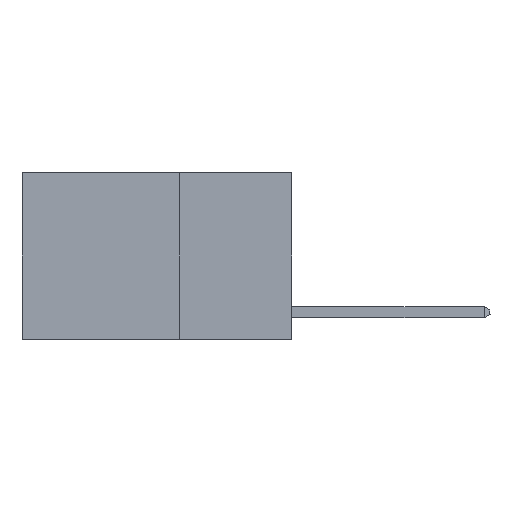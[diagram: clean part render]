
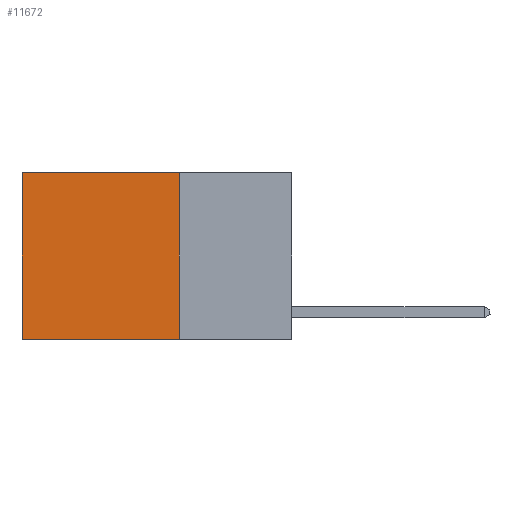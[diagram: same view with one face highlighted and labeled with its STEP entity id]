
A CAD part, left-side view. The second image highlights one B-rep face of the part: STEP entity #11672.
In plain terms, the highlighted planar face has unit normal (-1, 0, 0).
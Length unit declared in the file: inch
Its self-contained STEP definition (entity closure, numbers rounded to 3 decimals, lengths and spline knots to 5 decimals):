
#360 = VECTOR ( 'NONE', #8419, 39.37008 ) ;
#2024 = ORIENTED_EDGE ( 'NONE', *, *, #18143, .T. ) ;
#2514 = CARTESIAN_POINT ( 'NONE',  ( 0.2625, 0.6, -0.37 ) ) ;
#2698 = EDGE_LOOP ( 'NONE', ( #2024, #26090, #4861, #4713 ) ) ;
#2784 = VECTOR ( 'NONE', #22954, 39.37008 ) ;
#2805 = DIRECTION ( 'NONE',  ( 0., 0., -1. ) ) ;
#3324 = LINE ( 'NONE', #10023, #9294 ) ;
#4713 = ORIENTED_EDGE ( 'NONE', *, *, #6314, .T. ) ;
#4786 = VERTEX_POINT ( 'NONE', #8839 ) ;
#4861 = ORIENTED_EDGE ( 'NONE', *, *, #15027, .F. ) ;
#5280 = EDGE_CURVE ( 'NONE', #4786, #11597, #12227, .T. ) ;
#5562 = DIRECTION ( 'NONE',  ( 0., 0., -1. ) ) ;
#6314 = EDGE_CURVE ( 'NONE', #15035, #21700, #15975, .T. ) ;
#7137 = CARTESIAN_POINT ( 'NONE',  ( 0.2625, 0.6, 0. ) ) ;
#8419 = DIRECTION ( 'NONE',  ( 0., 1., 0. ) ) ;
#8839 = CARTESIAN_POINT ( 'NONE',  ( 0.2625, 0.25, -0.37 ) ) ;
#9294 = VECTOR ( 'NONE', #5562, 39.37008 ) ;
#10023 = CARTESIAN_POINT ( 'NONE',  ( 0.2625, 0.25, 0. ) ) ;
#10555 = CARTESIAN_POINT ( 'NONE',  ( 0.2625, 0.25, -0.37 ) ) ;
#11597 = VERTEX_POINT ( 'NONE', #2514 ) ;
#11658 = PLANE ( 'NONE',  #14629 ) ;
#11672 = ADVANCED_FACE ( 'NONE', ( #21176 ), #11658, .F. ) ;
#12227 = LINE ( 'NONE', #10555, #360 ) ;
#13778 = DIRECTION ( 'NONE',  ( 0., 0., -1. ) ) ;
#13918 = VECTOR ( 'NONE', #13778, 39.37008 ) ;
#14423 = CARTESIAN_POINT ( 'NONE',  ( 0.2625, 0.25, 0. ) ) ;
#14629 = AXIS2_PLACEMENT_3D ( 'NONE', #20441, #16089, #2805 ) ;
#15027 = EDGE_CURVE ( 'NONE', #15035, #4786, #3324, .T. ) ;
#15035 = VERTEX_POINT ( 'NONE', #14423 ) ;
#15975 = LINE ( 'NONE', #20713, #2784 ) ;
#16089 = DIRECTION ( 'NONE',  ( 1., 0., 0. ) ) ;
#17786 = CARTESIAN_POINT ( 'NONE',  ( 0.2625, 0.6, 0. ) ) ;
#18143 = EDGE_CURVE ( 'NONE', #21700, #11597, #19820, .T. ) ;
#19820 = LINE ( 'NONE', #7137, #13918 ) ;
#20441 = CARTESIAN_POINT ( 'NONE',  ( 0.2625, 0.25, 0. ) ) ;
#20713 = CARTESIAN_POINT ( 'NONE',  ( 0.2625, 0.25, 0. ) ) ;
#21176 = FACE_OUTER_BOUND ( 'NONE', #2698, .T. ) ;
#21700 = VERTEX_POINT ( 'NONE', #17786 ) ;
#22954 = DIRECTION ( 'NONE',  ( 0., 1., 0. ) ) ;
#26090 = ORIENTED_EDGE ( 'NONE', *, *, #5280, .F. ) ;
